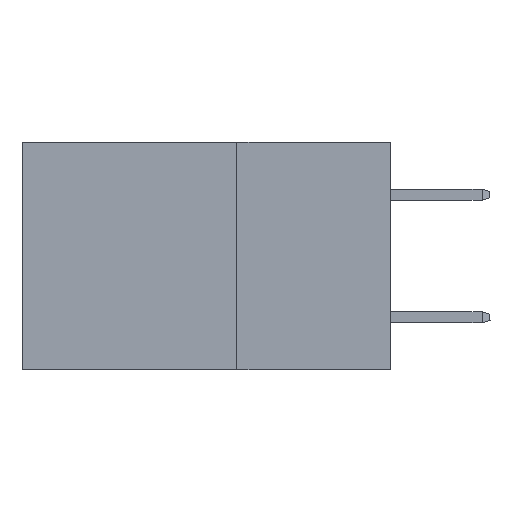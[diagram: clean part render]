
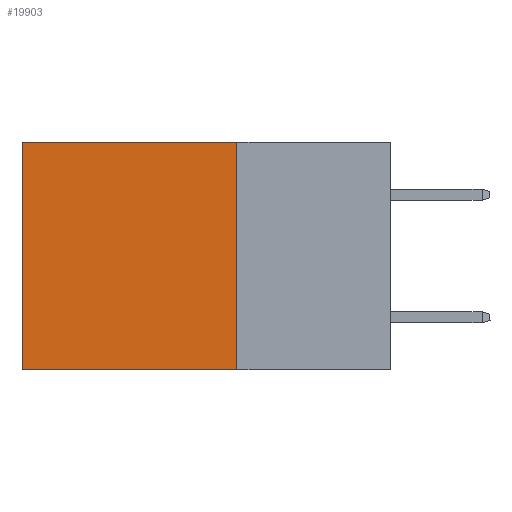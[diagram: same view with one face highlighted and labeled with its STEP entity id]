
A CAD part, left-side view. The second image highlights one B-rep face of the part: STEP entity #19903.
In plain terms, the highlighted planar face has unit normal (-1, 0, 0).
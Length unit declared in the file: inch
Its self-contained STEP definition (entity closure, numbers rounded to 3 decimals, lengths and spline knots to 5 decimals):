
#4785 = CARTESIAN_POINT ( 'NONE',  ( 0.2875, 0.6, 0. ) ) ;
#5580 = VECTOR ( 'NONE', #38140, 39.37008 ) ;
#6387 = EDGE_CURVE ( 'NONE', #30523, #25452, #11851, .T. ) ;
#8532 = ORIENTED_EDGE ( 'NONE', *, *, #6387, .F. ) ;
#8589 = DIRECTION ( 'NONE',  ( 0., 0., -1. ) ) ;
#8786 = PLANE ( 'NONE',  #30886 ) ;
#9743 = CARTESIAN_POINT ( 'NONE',  ( 0.2875, 0.25, 0. ) ) ;
#10814 = CARTESIAN_POINT ( 'NONE',  ( 0.2875, 0.25, 0. ) ) ;
#11851 = LINE ( 'NONE', #32813, #15180 ) ;
#11919 = ORIENTED_EDGE ( 'NONE', *, *, #20507, .F. ) ;
#12488 = EDGE_LOOP ( 'NONE', ( #16076, #8532, #11919, #26251 ) ) ;
#13424 = CARTESIAN_POINT ( 'NONE',  ( 0.2875, 0.25, -0.37 ) ) ;
#13748 = DIRECTION ( 'NONE',  ( 0., 0., -1. ) ) ;
#14437 = EDGE_CURVE ( 'NONE', #21129, #25452, #17378, .T. ) ;
#15180 = VECTOR ( 'NONE', #24010, 39.37008 ) ;
#16076 = ORIENTED_EDGE ( 'NONE', *, *, #14437, .T. ) ;
#16802 = EDGE_CURVE ( 'NONE', #29065, #21129, #27572, .T. ) ;
#17378 = LINE ( 'NONE', #22878, #5580 ) ;
#19903 = ADVANCED_FACE ( 'NONE', ( #29353 ), #8786, .F. ) ;
#20507 = EDGE_CURVE ( 'NONE', #29065, #30523, #28626, .T. ) ;
#21129 = VERTEX_POINT ( 'NONE', #4785 ) ;
#22682 = VECTOR ( 'NONE', #13748, 39.37008 ) ;
#22878 = CARTESIAN_POINT ( 'NONE',  ( 0.2875, 0.6, 0. ) ) ;
#23488 = DIRECTION ( 'NONE',  ( 1., 0., 0. ) ) ;
#24010 = DIRECTION ( 'NONE',  ( 0., 1., 0. ) ) ;
#25452 = VERTEX_POINT ( 'NONE', #30133 ) ;
#26251 = ORIENTED_EDGE ( 'NONE', *, *, #16802, .T. ) ;
#26418 = CARTESIAN_POINT ( 'NONE',  ( 0.2875, 0.25, 0. ) ) ;
#27572 = LINE ( 'NONE', #9743, #28181 ) ;
#28181 = VECTOR ( 'NONE', #30896, 39.37008 ) ;
#28626 = LINE ( 'NONE', #10814, #22682 ) ;
#29065 = VERTEX_POINT ( 'NONE', #30568 ) ;
#29353 = FACE_OUTER_BOUND ( 'NONE', #12488, .T. ) ;
#30133 = CARTESIAN_POINT ( 'NONE',  ( 0.2875, 0.6, -0.37 ) ) ;
#30523 = VERTEX_POINT ( 'NONE', #13424 ) ;
#30568 = CARTESIAN_POINT ( 'NONE',  ( 0.2875, 0.25, 0. ) ) ;
#30886 = AXIS2_PLACEMENT_3D ( 'NONE', #26418, #23488, #8589 ) ;
#30896 = DIRECTION ( 'NONE',  ( 0., 1., 0. ) ) ;
#32813 = CARTESIAN_POINT ( 'NONE',  ( 0.2875, 0.25, -0.37 ) ) ;
#38140 = DIRECTION ( 'NONE',  ( 0., 0., -1. ) ) ;
